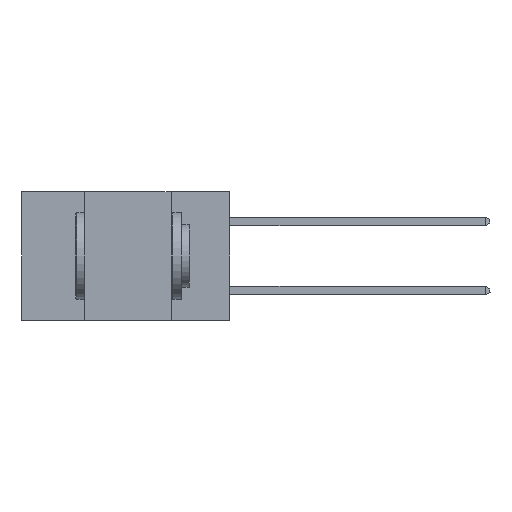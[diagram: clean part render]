
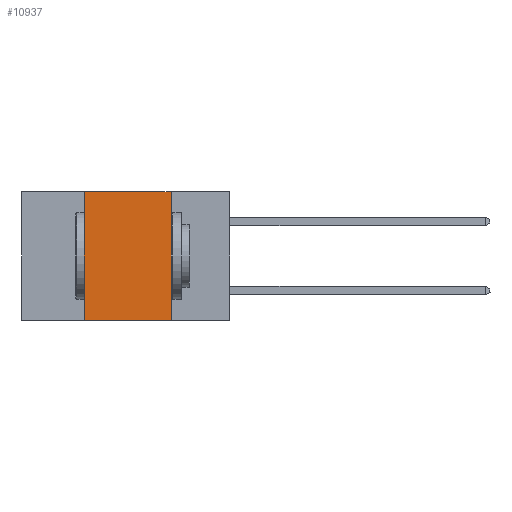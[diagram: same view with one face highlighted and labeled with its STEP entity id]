
A CAD part, left-side view. The second image highlights one B-rep face of the part: STEP entity #10937.
In plain terms, the highlighted planar face has unit normal (-1, 0, 0).
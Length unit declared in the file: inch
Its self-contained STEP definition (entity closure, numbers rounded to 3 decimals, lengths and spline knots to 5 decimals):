
#277 = EDGE_CURVE ( 'NONE', #1510, #15545, #16224, .T. ) ;
#1299 = CARTESIAN_POINT ( 'NONE',  ( 0., 0.6, 0. ) ) ;
#1369 = LINE ( 'NONE', #8486, #14832 ) ;
#1510 = VERTEX_POINT ( 'NONE', #3107 ) ;
#1663 = ORIENTED_EDGE ( 'NONE', *, *, #3879, .F. ) ;
#3107 = CARTESIAN_POINT ( 'NONE',  ( 0., 0.17, 0. ) ) ;
#3363 = CARTESIAN_POINT ( 'NONE',  ( 0., 0.42, -0.37 ) ) ;
#3879 = EDGE_CURVE ( 'NONE', #10665, #1510, #12458, .T. ) ;
#4448 = ORIENTED_EDGE ( 'NONE', *, *, #277, .F. ) ;
#4725 = CARTESIAN_POINT ( 'NONE',  ( 0., 0.42, 0. ) ) ;
#5374 = DIRECTION ( 'NONE',  ( 0., 0., -1. ) ) ;
#5821 = CARTESIAN_POINT ( 'NONE',  ( 0., 0.6, 0. ) ) ;
#6308 = CARTESIAN_POINT ( 'NONE',  ( 0., 0.42, 0. ) ) ;
#6701 = EDGE_LOOP ( 'NONE', ( #4448, #1663, #12759, #10218 ) ) ;
#7994 = VERTEX_POINT ( 'NONE', #3363 ) ;
#8469 = DIRECTION ( 'NONE',  ( 0., -1., 0. ) ) ;
#8486 = CARTESIAN_POINT ( 'NONE',  ( 0., 0.6, -0.37 ) ) ;
#8998 = EDGE_CURVE ( 'NONE', #7994, #15545, #1369, .T. ) ;
#9530 = DIRECTION ( 'NONE',  ( 1., 0., 0. ) ) ;
#9607 = CARTESIAN_POINT ( 'NONE',  ( 0., 0.17, -0.37 ) ) ;
#9852 = DIRECTION ( 'NONE',  ( 0., -1., 0. ) ) ;
#10218 = ORIENTED_EDGE ( 'NONE', *, *, #8998, .T. ) ;
#10665 = VERTEX_POINT ( 'NONE', #6308 ) ;
#10937 = ADVANCED_FACE ( 'NONE', ( #12418 ), #15012, .F. ) ;
#12418 = FACE_OUTER_BOUND ( 'NONE', #6701, .T. ) ;
#12458 = LINE ( 'NONE', #5821, #17381 ) ;
#12759 = ORIENTED_EDGE ( 'NONE', *, *, #14617, .F. ) ;
#13136 = VECTOR ( 'NONE', #14293, 39.37008 ) ;
#13731 = CARTESIAN_POINT ( 'NONE',  ( 0., 0.17, 0. ) ) ;
#13977 = LINE ( 'NONE', #4725, #13136 ) ;
#14293 = DIRECTION ( 'NONE',  ( 0., 0., 1. ) ) ;
#14617 = EDGE_CURVE ( 'NONE', #7994, #10665, #13977, .T. ) ;
#14832 = VECTOR ( 'NONE', #9852, 39.37008 ) ;
#15012 = PLANE ( 'NONE',  #15161 ) ;
#15161 = AXIS2_PLACEMENT_3D ( 'NONE', #1299, #9530, #17584 ) ;
#15545 = VERTEX_POINT ( 'NONE', #9607 ) ;
#15792 = VECTOR ( 'NONE', #5374, 39.37008 ) ;
#16224 = LINE ( 'NONE', #13731, #15792 ) ;
#17381 = VECTOR ( 'NONE', #8469, 39.37008 ) ;
#17584 = DIRECTION ( 'NONE',  ( 0., 0., -1. ) ) ;
